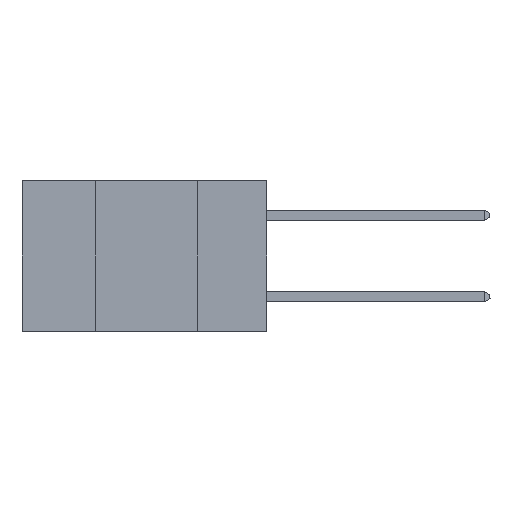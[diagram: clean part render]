
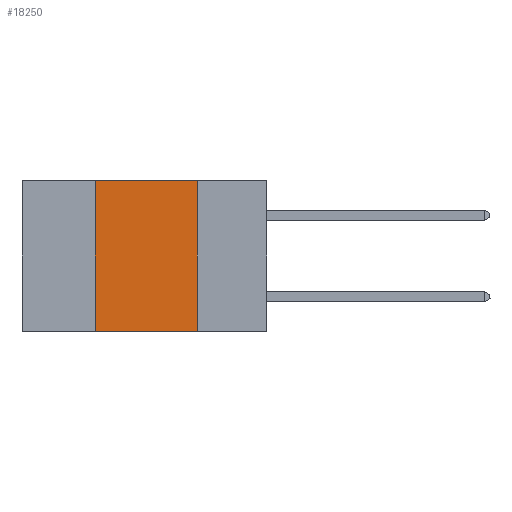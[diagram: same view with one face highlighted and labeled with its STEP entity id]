
A CAD part, left-side view. The second image highlights one B-rep face of the part: STEP entity #18250.
In plain terms, the highlighted planar face has unit normal (-1, 0, 0).
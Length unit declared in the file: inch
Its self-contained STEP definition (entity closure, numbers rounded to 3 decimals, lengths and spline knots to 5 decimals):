
#62 = LINE ( 'NONE', #23805, #3746 ) ;
#153 = VERTEX_POINT ( 'NONE', #914 ) ;
#914 = CARTESIAN_POINT ( 'NONE',  ( 0., 0.42, 0. ) ) ;
#917 = CARTESIAN_POINT ( 'NONE',  ( 0., 0.6, 0. ) ) ;
#1247 = DIRECTION ( 'NONE',  ( 0., 0., -1. ) ) ;
#1626 = ORIENTED_EDGE ( 'NONE', *, *, #8165, .F. ) ;
#2025 = LINE ( 'NONE', #3808, #30294 ) ;
#2459 = FACE_OUTER_BOUND ( 'NONE', #18813, .T. ) ;
#3746 = VECTOR ( 'NONE', #18899, 39.37008 ) ;
#3808 = CARTESIAN_POINT ( 'NONE',  ( 0., 0.17, 0. ) ) ;
#3977 = VERTEX_POINT ( 'NONE', #22978 ) ;
#4805 = DIRECTION ( 'NONE',  ( 0., 0., 1. ) ) ;
#5405 = VERTEX_POINT ( 'NONE', #29194 ) ;
#5693 = DIRECTION ( 'NONE',  ( 0., -1., 0. ) ) ;
#6532 = ORIENTED_EDGE ( 'NONE', *, *, #29600, .F. ) ;
#6543 = EDGE_CURVE ( 'NONE', #5405, #6876, #2025, .T. ) ;
#6876 = VERTEX_POINT ( 'NONE', #26679 ) ;
#8165 = EDGE_CURVE ( 'NONE', #3977, #153, #30187, .T. ) ;
#11144 = DIRECTION ( 'NONE',  ( 1., 0., 0. ) ) ;
#14514 = CARTESIAN_POINT ( 'NONE',  ( 0., 0.42, 0. ) ) ;
#15383 = CARTESIAN_POINT ( 'NONE',  ( 0., 0.6, -0.37 ) ) ;
#17783 = LINE ( 'NONE', #15383, #19941 ) ;
#17967 = DIRECTION ( 'NONE',  ( 0., 0., -1. ) ) ;
#18250 = ADVANCED_FACE ( 'NONE', ( #2459 ), #29075, .F. ) ;
#18813 = EDGE_LOOP ( 'NONE', ( #27672, #6532, #1626, #23887 ) ) ;
#18899 = DIRECTION ( 'NONE',  ( 0., -1., 0. ) ) ;
#19941 = VECTOR ( 'NONE', #5693, 39.37008 ) ;
#22978 = CARTESIAN_POINT ( 'NONE',  ( 0., 0.42, -0.37 ) ) ;
#23627 = AXIS2_PLACEMENT_3D ( 'NONE', #917, #11144, #1247 ) ;
#23805 = CARTESIAN_POINT ( 'NONE',  ( 0., 0.6, 0. ) ) ;
#23887 = ORIENTED_EDGE ( 'NONE', *, *, #27716, .T. ) ;
#26679 = CARTESIAN_POINT ( 'NONE',  ( 0., 0.17, -0.37 ) ) ;
#27672 = ORIENTED_EDGE ( 'NONE', *, *, #6543, .F. ) ;
#27716 = EDGE_CURVE ( 'NONE', #3977, #6876, #17783, .T. ) ;
#29075 = PLANE ( 'NONE',  #23627 ) ;
#29194 = CARTESIAN_POINT ( 'NONE',  ( 0., 0.17, 0. ) ) ;
#29431 = VECTOR ( 'NONE', #4805, 39.37008 ) ;
#29600 = EDGE_CURVE ( 'NONE', #153, #5405, #62, .T. ) ;
#30187 = LINE ( 'NONE', #14514, #29431 ) ;
#30294 = VECTOR ( 'NONE', #17967, 39.37008 ) ;
